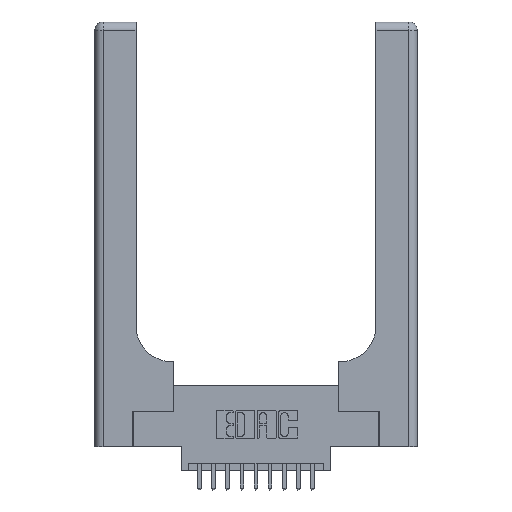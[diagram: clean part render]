
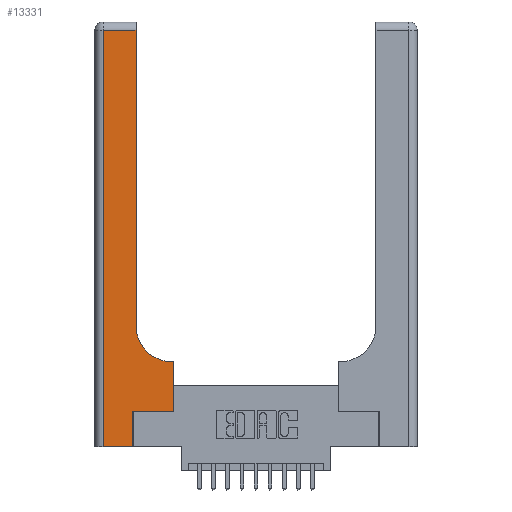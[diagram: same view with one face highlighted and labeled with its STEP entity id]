
A CAD part, top view. The second image highlights one B-rep face of the part: STEP entity #13331.
In plain terms, the highlighted planar face has unit normal (0, 0, 1).
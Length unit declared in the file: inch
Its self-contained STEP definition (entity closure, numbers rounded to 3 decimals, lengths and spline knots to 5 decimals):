
#78 = PLANE ( 'NONE',  #12801 ) ;
#270 = LINE ( 'NONE', #788, #4587 ) ;
#657 = EDGE_CURVE ( 'NONE', #10632, #5454, #832, .T. ) ;
#663 = CARTESIAN_POINT ( 'NONE',  ( 0.06, 0., 0.37 ) ) ;
#788 = CARTESIAN_POINT ( 'NONE',  ( 0.2915, 3., 0.37 ) ) ;
#832 = LINE ( 'NONE', #1969, #3928 ) ;
#1027 = VECTOR ( 'NONE', #9171, 39.37008 ) ;
#1059 = EDGE_CURVE ( 'NONE', #5454, #7805, #4955, .T. ) ;
#1243 = DIRECTION ( 'NONE',  ( 1., 0., 0. ) ) ;
#1724 = VECTOR ( 'NONE', #5202, 39.37008 ) ;
#1859 = VERTEX_POINT ( 'NONE', #4142 ) ;
#1969 = CARTESIAN_POINT ( 'NONE',  ( 0., 0., 0.37 ) ) ;
#2588 = CARTESIAN_POINT ( 'NONE',  ( 0.269, 0., 0.37 ) ) ;
#3306 = ORIENTED_EDGE ( 'NONE', *, *, #7331, .T. ) ;
#3481 = CARTESIAN_POINT ( 'NONE',  ( 0.5585, 0.25, 0.37 ) ) ;
#3928 = VECTOR ( 'NONE', #10981, 39.37008 ) ;
#4055 = EDGE_LOOP ( 'NONE', ( #6642, #5822, #10978, #16158, #9378, #3306, #8975, #11974, #7446 ) ) ;
#4133 = VECTOR ( 'NONE', #13176, 39.37008 ) ;
#4142 = CARTESIAN_POINT ( 'NONE',  ( 0.5415, 0.6, 0.37 ) ) ;
#4587 = VECTOR ( 'NONE', #16184, 39.37008 ) ;
#4590 = CARTESIAN_POINT ( 'NONE',  ( 0.269, 0.25, 0.37 ) ) ;
#4637 = VERTEX_POINT ( 'NONE', #3481 ) ;
#4955 = LINE ( 'NONE', #2588, #1027 ) ;
#5202 = DIRECTION ( 'NONE',  ( -1., 0., 0. ) ) ;
#5454 = VERTEX_POINT ( 'NONE', #15566 ) ;
#5822 = ORIENTED_EDGE ( 'NONE', *, *, #9483, .T. ) ;
#6642 = ORIENTED_EDGE ( 'NONE', *, *, #8006, .T. ) ;
#6913 = VERTEX_POINT ( 'NONE', #10412 ) ;
#7331 = EDGE_CURVE ( 'NONE', #7805, #4637, #7589, .T. ) ;
#7392 = AXIS2_PLACEMENT_3D ( 'NONE', #9053, #16828, #1243 ) ;
#7446 = ORIENTED_EDGE ( 'NONE', *, *, #15953, .T. ) ;
#7581 = LINE ( 'NONE', #10464, #4133 ) ;
#7589 = LINE ( 'NONE', #4590, #7774 ) ;
#7652 = LINE ( 'NONE', #16791, #1724 ) ;
#7680 = CARTESIAN_POINT ( 'NONE',  ( 0.5585, 0.6, 0.37 ) ) ;
#7746 = LINE ( 'NONE', #11089, #13808 ) ;
#7774 = VECTOR ( 'NONE', #14985, 39.37008 ) ;
#7805 = VERTEX_POINT ( 'NONE', #12326 ) ;
#8006 = EDGE_CURVE ( 'NONE', #15261, #6913, #270, .T. ) ;
#8975 = ORIENTED_EDGE ( 'NONE', *, *, #10187, .T. ) ;
#9053 = CARTESIAN_POINT ( 'NONE',  ( 0.5415, 0.85, 0.37 ) ) ;
#9171 = DIRECTION ( 'NONE',  ( 0., 1., 0. ) ) ;
#9378 = ORIENTED_EDGE ( 'NONE', *, *, #1059, .T. ) ;
#9483 = EDGE_CURVE ( 'NONE', #6913, #15839, #7581, .T. ) ;
#9966 = DIRECTION ( 'NONE',  ( 0., 1., 0. ) ) ;
#10187 = EDGE_CURVE ( 'NONE', #4637, #14803, #7746, .T. ) ;
#10412 = CARTESIAN_POINT ( 'NONE',  ( 0.2915, 2.94, 0.37 ) ) ;
#10464 = CARTESIAN_POINT ( 'NONE',  ( 0., 2.94, 0.37 ) ) ;
#10632 = VERTEX_POINT ( 'NONE', #663 ) ;
#10704 = VECTOR ( 'NONE', #15587, 39.37008 ) ;
#10978 = ORIENTED_EDGE ( 'NONE', *, *, #11784, .T. ) ;
#10981 = DIRECTION ( 'NONE',  ( 1., 0., 0. ) ) ;
#11089 = CARTESIAN_POINT ( 'NONE',  ( 0.5585, 0.25, 0.37 ) ) ;
#11481 = CARTESIAN_POINT ( 'NONE',  ( 0., 3., 0.37 ) ) ;
#11784 = EDGE_CURVE ( 'NONE', #15839, #10632, #16403, .T. ) ;
#11974 = ORIENTED_EDGE ( 'NONE', *, *, #13353, .T. ) ;
#12326 = CARTESIAN_POINT ( 'NONE',  ( 0.269, 0.25, 0.37 ) ) ;
#12706 = CARTESIAN_POINT ( 'NONE',  ( 0.06, 2.94, 0.37 ) ) ;
#12786 = DIRECTION ( 'NONE',  ( 0., 0., -1. ) ) ;
#12801 = AXIS2_PLACEMENT_3D ( 'NONE', #11481, #12786, #16851 ) ;
#13176 = DIRECTION ( 'NONE',  ( -1., 0., 0. ) ) ;
#13331 = ADVANCED_FACE ( 'NONE', ( #15749 ), #78, .F. ) ;
#13353 = EDGE_CURVE ( 'NONE', #14803, #1859, #7652, .T. ) ;
#13808 = VECTOR ( 'NONE', #9966, 39.37008 ) ;
#14159 = CARTESIAN_POINT ( 'NONE',  ( 0.06, 3., 0.37 ) ) ;
#14375 = CIRCLE ( 'NONE', #7392, 0.25 ) ;
#14803 = VERTEX_POINT ( 'NONE', #7680 ) ;
#14985 = DIRECTION ( 'NONE',  ( 1., 0., 0. ) ) ;
#15261 = VERTEX_POINT ( 'NONE', #16736 ) ;
#15566 = CARTESIAN_POINT ( 'NONE',  ( 0.269, 0., 0.37 ) ) ;
#15587 = DIRECTION ( 'NONE',  ( 0., -1., 0. ) ) ;
#15749 = FACE_OUTER_BOUND ( 'NONE', #4055, .T. ) ;
#15839 = VERTEX_POINT ( 'NONE', #12706 ) ;
#15953 = EDGE_CURVE ( 'NONE', #1859, #15261, #14375, .T. ) ;
#16158 = ORIENTED_EDGE ( 'NONE', *, *, #657, .T. ) ;
#16184 = DIRECTION ( 'NONE',  ( 0., 1., 0. ) ) ;
#16403 = LINE ( 'NONE', #14159, #10704 ) ;
#16736 = CARTESIAN_POINT ( 'NONE',  ( 0.2915, 0.85, 0.37 ) ) ;
#16791 = CARTESIAN_POINT ( 'NONE',  ( 0.2915, 0.6, 0.37 ) ) ;
#16828 = DIRECTION ( 'NONE',  ( 0., 0., -1. ) ) ;
#16851 = DIRECTION ( 'NONE',  ( -1., 0., 0. ) ) ;
